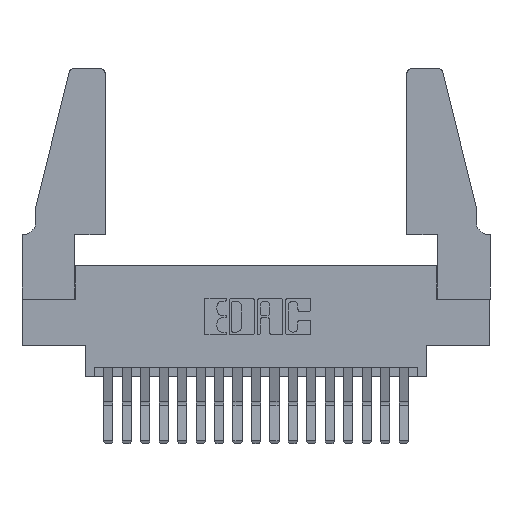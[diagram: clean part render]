
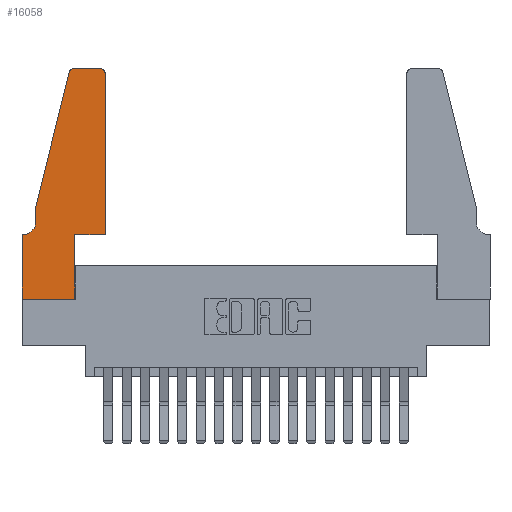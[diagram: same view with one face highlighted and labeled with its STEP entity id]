
A CAD part, top view. The second image highlights one B-rep face of the part: STEP entity #16058.
In plain terms, the highlighted planar face has unit normal (0, 0, 1).
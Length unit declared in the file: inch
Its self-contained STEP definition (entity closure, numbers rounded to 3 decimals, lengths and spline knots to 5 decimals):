
#226 = CARTESIAN_POINT ( 'NONE',  ( 0.2865, 0., 0.37 ) ) ;
#239 = EDGE_CURVE ( 'NONE', #8017, #11733, #10090, .T. ) ;
#498 = VECTOR ( 'NONE', #18631, 39.37008 ) ;
#522 = LINE ( 'NONE', #14555, #8116 ) ;
#2138 = DIRECTION ( 'NONE',  ( 0., 0., -1. ) ) ;
#2274 = VERTEX_POINT ( 'NONE', #10764 ) ;
#2340 = CARTESIAN_POINT ( 'NONE',  ( 0., 0.35, 0.37 ) ) ;
#2424 = CARTESIAN_POINT ( 'NONE',  ( 0.2605, 1.25, 0.37 ) ) ;
#2481 = EDGE_CURVE ( 'NONE', #11733, #9576, #5888, .T. ) ;
#2491 = DIRECTION ( 'NONE',  ( -1., 0., 0. ) ) ;
#2579 = CIRCLE ( 'NONE', #11043, 0.03 ) ;
#3068 = VERTEX_POINT ( 'NONE', #18446 ) ;
#3198 = CARTESIAN_POINT ( 'NONE',  ( 0., 0.35, 0.37 ) ) ;
#3292 = EDGE_LOOP ( 'NONE', ( #10539, #3341, #18795, #16387, #8059, #13089, #5065, #4637, #12468, #12721, #10925, #4721 ) ) ;
#3336 = AXIS2_PLACEMENT_3D ( 'NONE', #6155, #6137, #6111 ) ;
#3341 = ORIENTED_EDGE ( 'NONE', *, *, #2481, .T. ) ;
#3427 = CARTESIAN_POINT ( 'NONE',  ( 0.0055, 0.35, 0.37 ) ) ;
#3902 = DIRECTION ( 'NONE',  ( 0., 0., 1. ) ) ;
#4190 = VERTEX_POINT ( 'NONE', #226 ) ;
#4547 = DIRECTION ( 'NONE',  ( 0., 1., 0. ) ) ;
#4637 = ORIENTED_EDGE ( 'NONE', *, *, #8913, .T. ) ;
#4721 = ORIENTED_EDGE ( 'NONE', *, *, #8367, .T. ) ;
#5065 = ORIENTED_EDGE ( 'NONE', *, *, #5120, .T. ) ;
#5120 = EDGE_CURVE ( 'NONE', #17772, #3068, #14267, .T. ) ;
#5232 = EDGE_CURVE ( 'NONE', #11450, #17772, #12460, .T. ) ;
#5562 = EDGE_CURVE ( 'NONE', #9576, #14013, #18030, .T. ) ;
#5647 = CARTESIAN_POINT ( 'NONE',  ( 0.4505, 0.35, 0.37 ) ) ;
#5888 = CIRCLE ( 'NONE', #3336, 0.03 ) ;
#5942 = VERTEX_POINT ( 'NONE', #9960 ) ;
#6106 = EDGE_CURVE ( 'NONE', #4190, #5942, #12897, .T. ) ;
#6111 = DIRECTION ( 'NONE',  ( 1., 0., 0. ) ) ;
#6137 = DIRECTION ( 'NONE',  ( 0., 0., 1. ) ) ;
#6155 = CARTESIAN_POINT ( 'NONE',  ( 0.284, 1.22, 0.37 ) ) ;
#6914 = CARTESIAN_POINT ( 'NONE',  ( 0., 0., 0.37 ) ) ;
#7316 = DIRECTION ( 'NONE',  ( 1., 0., 0. ) ) ;
#7533 = VECTOR ( 'NONE', #14383, 39.37008 ) ;
#7981 = VERTEX_POINT ( 'NONE', #8856 ) ;
#8017 = VERTEX_POINT ( 'NONE', #10418 ) ;
#8059 = ORIENTED_EDGE ( 'NONE', *, *, #8995, .T. ) ;
#8116 = VECTOR ( 'NONE', #7316, 39.37008 ) ;
#8259 = DIRECTION ( 'NONE',  ( 0., 0., 1. ) ) ;
#8367 = EDGE_CURVE ( 'NONE', #2274, #8017, #2579, .T. ) ;
#8572 = CARTESIAN_POINT ( 'NONE',  ( 0.0755, 0.42, 0.37 ) ) ;
#8856 = CARTESIAN_POINT ( 'NONE',  ( 0.4505, 0.35, 0.37 ) ) ;
#8913 = EDGE_CURVE ( 'NONE', #3068, #4190, #11616, .T. ) ;
#8921 = CARTESIAN_POINT ( 'NONE',  ( 0.2865, 0.35, 0.37 ) ) ;
#8989 = VECTOR ( 'NONE', #4547, 39.37008 ) ;
#8995 = EDGE_CURVE ( 'NONE', #16167, #11450, #17455, .T. ) ;
#9576 = VERTEX_POINT ( 'NONE', #13743 ) ;
#9904 = CARTESIAN_POINT ( 'NONE',  ( 0.284, 1.25, 0.37 ) ) ;
#9960 = CARTESIAN_POINT ( 'NONE',  ( 0.2865, 0.35, 0.37 ) ) ;
#10090 = LINE ( 'NONE', #2424, #17293 ) ;
#10328 = AXIS2_PLACEMENT_3D ( 'NONE', #11084, #2138, #12546 ) ;
#10418 = CARTESIAN_POINT ( 'NONE',  ( 0.4205, 1.25, 0.37 ) ) ;
#10539 = ORIENTED_EDGE ( 'NONE', *, *, #239, .T. ) ;
#10670 = DIRECTION ( 'NONE',  ( -0.239, -0.971, 0. ) ) ;
#10764 = CARTESIAN_POINT ( 'NONE',  ( 0.4505, 1.22, 0.37 ) ) ;
#10925 = ORIENTED_EDGE ( 'NONE', *, *, #14181, .T. ) ;
#11043 = AXIS2_PLACEMENT_3D ( 'NONE', #16916, #8259, #18351 ) ;
#11084 = CARTESIAN_POINT ( 'NONE',  ( 0.0055, 0.42, 0.37 ) ) ;
#11261 = PLANE ( 'NONE',  #14983 ) ;
#11291 = DIRECTION ( 'NONE',  ( 0., -1., 0. ) ) ;
#11450 = VERTEX_POINT ( 'NONE', #3427 ) ;
#11616 = LINE ( 'NONE', #15166, #18325 ) ;
#11733 = VERTEX_POINT ( 'NONE', #9904 ) ;
#12015 = FACE_OUTER_BOUND ( 'NONE', #3292, .T. ) ;
#12363 = DIRECTION ( 'NONE',  ( 1., 0., 0. ) ) ;
#12460 = LINE ( 'NONE', #17194, #498 ) ;
#12468 = ORIENTED_EDGE ( 'NONE', *, *, #6106, .T. ) ;
#12546 = DIRECTION ( 'NONE',  ( -1., 0., 0. ) ) ;
#12721 = ORIENTED_EDGE ( 'NONE', *, *, #16233, .T. ) ;
#12897 = LINE ( 'NONE', #8921, #8989 ) ;
#13089 = ORIENTED_EDGE ( 'NONE', *, *, #5232, .T. ) ;
#13532 = CARTESIAN_POINT ( 'NONE',  ( 0.0755, 0.5, 0.37 ) ) ;
#13743 = CARTESIAN_POINT ( 'NONE',  ( 0.25487, 1.22718, 0.37 ) ) ;
#13954 = CARTESIAN_POINT ( 'NONE',  ( 0.0755, 0.5, 0.37 ) ) ;
#14013 = VERTEX_POINT ( 'NONE', #13954 ) ;
#14181 = EDGE_CURVE ( 'NONE', #7981, #2274, #18129, .T. ) ;
#14189 = DIRECTION ( 'NONE',  ( 1., 0., 0. ) ) ;
#14251 = VECTOR ( 'NONE', #10670, 39.37008 ) ;
#14267 = LINE ( 'NONE', #6914, #18044 ) ;
#14383 = DIRECTION ( 'NONE',  ( 0., 1., 0. ) ) ;
#14555 = CARTESIAN_POINT ( 'NONE',  ( 0.4505, 0.35, 0.37 ) ) ;
#14687 = CARTESIAN_POINT ( 'NONE',  ( 0.0755, 0.5, 0.37 ) ) ;
#14983 = AXIS2_PLACEMENT_3D ( 'NONE', #2340, #3902, #14189 ) ;
#15079 = LINE ( 'NONE', #14687, #17979 ) ;
#15166 = CARTESIAN_POINT ( 'NONE',  ( 0., 0., 0.37 ) ) ;
#16058 = ADVANCED_FACE ( 'NONE', ( #12015 ), #11261, .T. ) ;
#16109 = DIRECTION ( 'NONE',  ( 0., -1., 0. ) ) ;
#16167 = VERTEX_POINT ( 'NONE', #8572 ) ;
#16233 = EDGE_CURVE ( 'NONE', #5942, #7981, #522, .T. ) ;
#16387 = ORIENTED_EDGE ( 'NONE', *, *, #18279, .T. ) ;
#16916 = CARTESIAN_POINT ( 'NONE',  ( 0.4205, 1.22, 0.37 ) ) ;
#17194 = CARTESIAN_POINT ( 'NONE',  ( 0.0755, 0.35, 0.37 ) ) ;
#17293 = VECTOR ( 'NONE', #2491, 39.37008 ) ;
#17455 = CIRCLE ( 'NONE', #10328, 0.07 ) ;
#17772 = VERTEX_POINT ( 'NONE', #3198 ) ;
#17979 = VECTOR ( 'NONE', #16109, 39.37008 ) ;
#18030 = LINE ( 'NONE', #13532, #14251 ) ;
#18044 = VECTOR ( 'NONE', #11291, 39.37008 ) ;
#18129 = LINE ( 'NONE', #5647, #7533 ) ;
#18279 = EDGE_CURVE ( 'NONE', #14013, #16167, #15079, .T. ) ;
#18325 = VECTOR ( 'NONE', #12363, 39.37008 ) ;
#18351 = DIRECTION ( 'NONE',  ( 1., 0., 0. ) ) ;
#18446 = CARTESIAN_POINT ( 'NONE',  ( 0., 0., 0.37 ) ) ;
#18631 = DIRECTION ( 'NONE',  ( -1., 0., 0. ) ) ;
#18795 = ORIENTED_EDGE ( 'NONE', *, *, #5562, .T. ) ;
